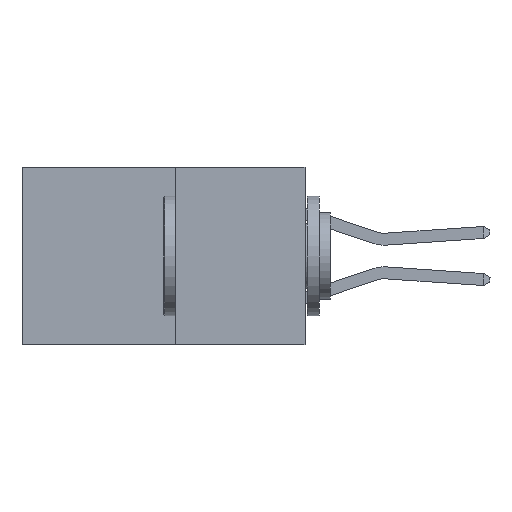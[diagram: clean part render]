
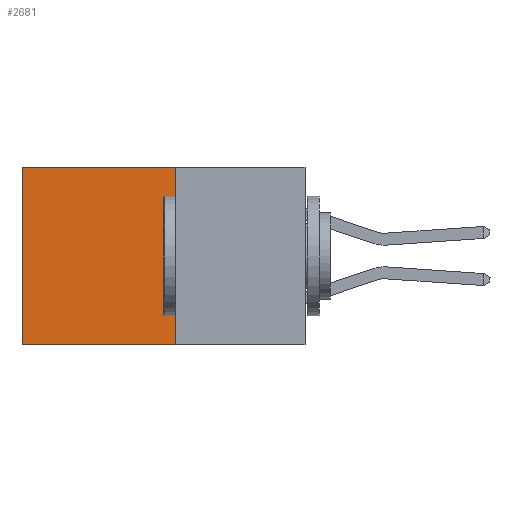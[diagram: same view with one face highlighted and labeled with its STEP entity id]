
A CAD part, left-side view. The second image highlights one B-rep face of the part: STEP entity #2681.
In plain terms, the highlighted planar face has unit normal (-1, 0, 0).
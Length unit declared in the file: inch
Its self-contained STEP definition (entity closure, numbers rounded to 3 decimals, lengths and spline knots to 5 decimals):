
#432 = ORIENTED_EDGE ( 'NONE', *, *, #2110, .F. ) ;
#447 = VECTOR ( 'NONE', #5292, 39.37008 ) ;
#1371 = LINE ( 'NONE', #5390, #447 ) ;
#2025 = CARTESIAN_POINT ( 'NONE',  ( 0.277, 0.27, 0. ) ) ;
#2110 = EDGE_CURVE ( 'NONE', #6246, #2400, #6560, .T. ) ;
#2400 = VERTEX_POINT ( 'NONE', #7345 ) ;
#2681 = ADVANCED_FACE ( 'NONE', ( #8944 ), #6005, .F. ) ;
#2939 = EDGE_LOOP ( 'NONE', ( #4807, #5431, #432, #9015 ) ) ;
#3170 = CARTESIAN_POINT ( 'NONE',  ( 0.277, 0.59, 0. ) ) ;
#3239 = DIRECTION ( 'NONE',  ( 0., 0., -1. ) ) ;
#3548 = AXIS2_PLACEMENT_3D ( 'NONE', #9707, #10902, #10805 ) ;
#3869 = VECTOR ( 'NONE', #10734, 39.37008 ) ;
#3950 = VERTEX_POINT ( 'NONE', #7458 ) ;
#4105 = LINE ( 'NONE', #7530, #9110 ) ;
#4194 = LINE ( 'NONE', #7205, #9188 ) ;
#4807 = ORIENTED_EDGE ( 'NONE', *, *, #8920, .T. ) ;
#5292 = DIRECTION ( 'NONE',  ( 0., 1., 0. ) ) ;
#5390 = CARTESIAN_POINT ( 'NONE',  ( 0.277, 0.27, -0.37 ) ) ;
#5431 = ORIENTED_EDGE ( 'NONE', *, *, #5921, .F. ) ;
#5763 = EDGE_CURVE ( 'NONE', #6246, #7569, #4194, .T. ) ;
#5921 = EDGE_CURVE ( 'NONE', #2400, #3950, #1371, .T. ) ;
#6005 = PLANE ( 'NONE',  #3548 ) ;
#6246 = VERTEX_POINT ( 'NONE', #2025 ) ;
#6560 = LINE ( 'NONE', #11139, #3869 ) ;
#7205 = CARTESIAN_POINT ( 'NONE',  ( 0.277, 0.27, 0. ) ) ;
#7322 = DIRECTION ( 'NONE',  ( 0., 1., 0. ) ) ;
#7345 = CARTESIAN_POINT ( 'NONE',  ( 0.277, 0.27, -0.37 ) ) ;
#7458 = CARTESIAN_POINT ( 'NONE',  ( 0.277, 0.59, -0.37 ) ) ;
#7530 = CARTESIAN_POINT ( 'NONE',  ( 0.277, 0.59, -0.37 ) ) ;
#7569 = VERTEX_POINT ( 'NONE', #3170 ) ;
#8920 = EDGE_CURVE ( 'NONE', #7569, #3950, #4105, .T. ) ;
#8944 = FACE_OUTER_BOUND ( 'NONE', #2939, .T. ) ;
#9015 = ORIENTED_EDGE ( 'NONE', *, *, #5763, .T. ) ;
#9110 = VECTOR ( 'NONE', #3239, 39.37008 ) ;
#9188 = VECTOR ( 'NONE', #7322, 39.37008 ) ;
#9707 = CARTESIAN_POINT ( 'NONE',  ( 0.277, 0.27, -0.37 ) ) ;
#10734 = DIRECTION ( 'NONE',  ( 0., 0., -1. ) ) ;
#10805 = DIRECTION ( 'NONE',  ( 0., 0., -1. ) ) ;
#10902 = DIRECTION ( 'NONE',  ( 1., 0., 0. ) ) ;
#11139 = CARTESIAN_POINT ( 'NONE',  ( 0.277, 0.27, -0.37 ) ) ;
